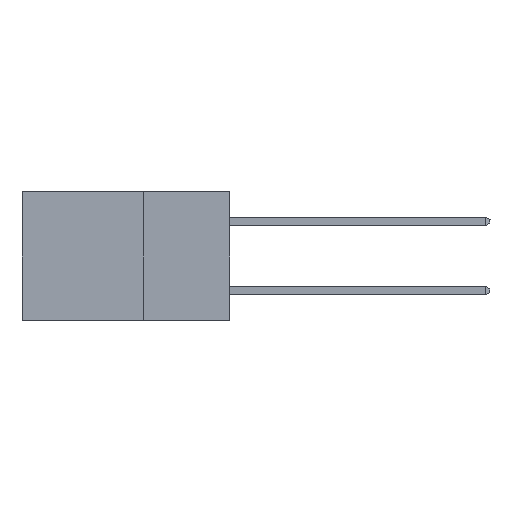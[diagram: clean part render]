
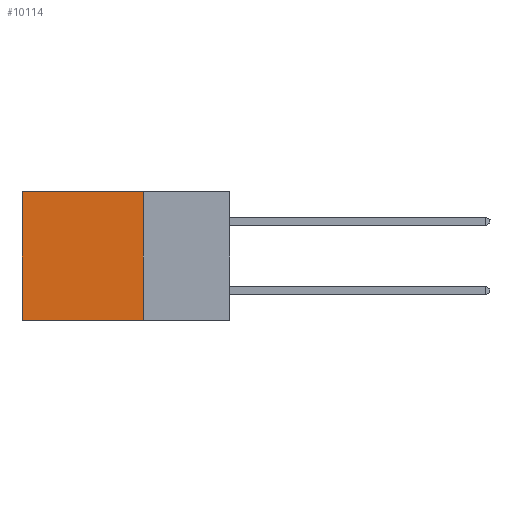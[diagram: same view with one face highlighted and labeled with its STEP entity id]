
A CAD part, left-side view. The second image highlights one B-rep face of the part: STEP entity #10114.
In plain terms, the highlighted planar face has unit normal (-1, 0, 0).
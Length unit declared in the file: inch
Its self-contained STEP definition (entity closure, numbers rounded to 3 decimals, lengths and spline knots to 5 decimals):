
#81 = EDGE_LOOP ( 'NONE', ( #746, #1089, #7698, #7652 ) ) ;
#381 = VERTEX_POINT ( 'NONE', #1390 ) ;
#466 = DIRECTION ( 'NONE',  ( 0., 0., -1. ) ) ;
#746 = ORIENTED_EDGE ( 'NONE', *, *, #13378, .T. ) ;
#1089 = ORIENTED_EDGE ( 'NONE', *, *, #11583, .F. ) ;
#1390 = CARTESIAN_POINT ( 'NONE',  ( 0.2615, 0.25, 0. ) ) ;
#1702 = LINE ( 'NONE', #12512, #13246 ) ;
#2404 = CARTESIAN_POINT ( 'NONE',  ( 0.2615, 0.25, -0.37 ) ) ;
#2543 = VERTEX_POINT ( 'NONE', #13435 ) ;
#2646 = CARTESIAN_POINT ( 'NONE',  ( 0.2615, 0.6, -0.37 ) ) ;
#2699 = EDGE_CURVE ( 'NONE', #381, #13076, #1702, .T. ) ;
#4167 = PLANE ( 'NONE',  #4217 ) ;
#4217 = AXIS2_PLACEMENT_3D ( 'NONE', #9487, #5251, #12795 ) ;
#4974 = VECTOR ( 'NONE', #466, 39.37008 ) ;
#5041 = DIRECTION ( 'NONE',  ( 0., 1., 0. ) ) ;
#5251 = DIRECTION ( 'NONE',  ( 1., 0., 0. ) ) ;
#5387 = VERTEX_POINT ( 'NONE', #2646 ) ;
#5669 = VECTOR ( 'NONE', #10138, 39.37008 ) ;
#7403 = FACE_OUTER_BOUND ( 'NONE', #81, .T. ) ;
#7652 = ORIENTED_EDGE ( 'NONE', *, *, #2699, .T. ) ;
#7698 = ORIENTED_EDGE ( 'NONE', *, *, #9419, .F. ) ;
#8761 = CARTESIAN_POINT ( 'NONE',  ( 0.2615, 0.25, -0.37 ) ) ;
#9008 = DIRECTION ( 'NONE',  ( 0., 0., -1. ) ) ;
#9380 = CARTESIAN_POINT ( 'NONE',  ( 0.2615, 0.6, -0.37 ) ) ;
#9419 = EDGE_CURVE ( 'NONE', #381, #2543, #10021, .T. ) ;
#9487 = CARTESIAN_POINT ( 'NONE',  ( 0.2615, 0.25, -0.37 ) ) ;
#10021 = LINE ( 'NONE', #2404, #10163 ) ;
#10114 = ADVANCED_FACE ( 'NONE', ( #7403 ), #4167, .F. ) ;
#10138 = DIRECTION ( 'NONE',  ( 0., 1., 0. ) ) ;
#10163 = VECTOR ( 'NONE', #9008, 39.37008 ) ;
#10687 = CARTESIAN_POINT ( 'NONE',  ( 0.2615, 0.6, 0. ) ) ;
#10919 = LINE ( 'NONE', #8761, #5669 ) ;
#11541 = LINE ( 'NONE', #9380, #4974 ) ;
#11583 = EDGE_CURVE ( 'NONE', #2543, #5387, #10919, .T. ) ;
#12512 = CARTESIAN_POINT ( 'NONE',  ( 0.2615, 0.25, 0. ) ) ;
#12795 = DIRECTION ( 'NONE',  ( 0., 0., -1. ) ) ;
#13076 = VERTEX_POINT ( 'NONE', #10687 ) ;
#13246 = VECTOR ( 'NONE', #5041, 39.37008 ) ;
#13378 = EDGE_CURVE ( 'NONE', #13076, #5387, #11541, .T. ) ;
#13435 = CARTESIAN_POINT ( 'NONE',  ( 0.2615, 0.25, -0.37 ) ) ;
